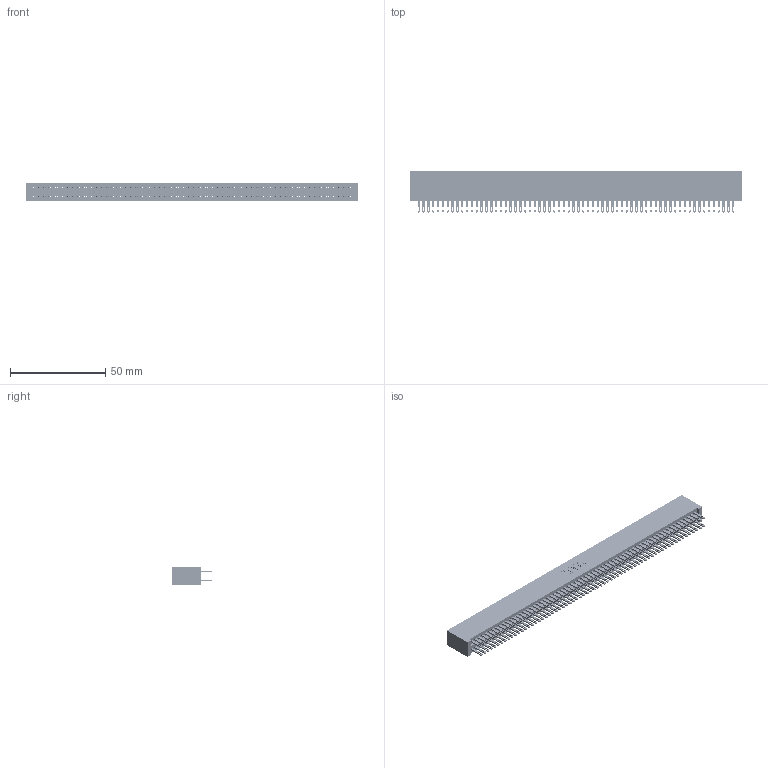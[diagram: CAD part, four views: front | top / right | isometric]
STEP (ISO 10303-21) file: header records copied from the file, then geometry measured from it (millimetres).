
FILE_DESCRIPTION (( 'STEP AP203' ), '1' );
FILE_NAME ('345-132-500-201.STEP', '2018-10-20T02:49:44', ( '' ), ( '' ), 'SwSTEP 2.0', 'SolidWorks 2016', '' );
FILE_SCHEMA (( 'CONFIG_CONTROL_DESIGN' ));
Length unit declared in the file: inch
Products named in the file (3): 345-132-500-201; 345 Part_No Mounting Lugs; 345-292-001_345-293-100
Assembly tree (133 placements, depth 2):
  345-132-500-201
    345 Part_No Mounting Lugs
    345-292-001_345-293-100  x132
Bounding box: 174.24 x 21.51 x 9.4 mm (x, y, z)
Volume: 18168.3 mm3; surface area: 28970.2 mm2
Topology: 133 solids, 133 shells, 6190 faces, 18929 edges, 12618 vertices
Faces by surface type: plane 3640, cylinder 2550
Entity records: 48207 total; most frequent: CARTESIAN_POINT 8056, ORIENTED_EDGE 7990, DIRECTION 7071, EDGE_CURVE 3995, LINE 3603, VECTOR 3603, VERTEX_POINT 2662, AXIS2_PLACEMENT_3D 1734
